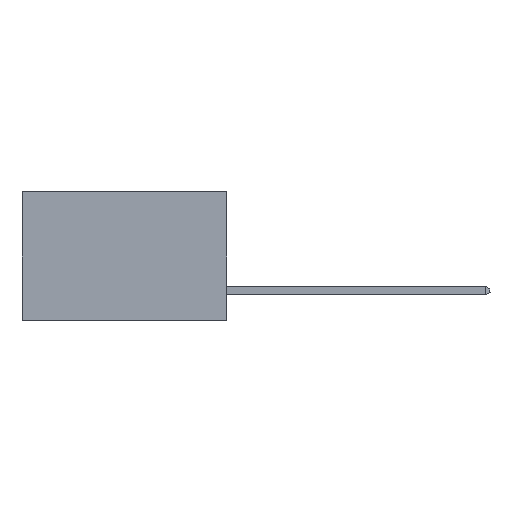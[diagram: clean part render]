
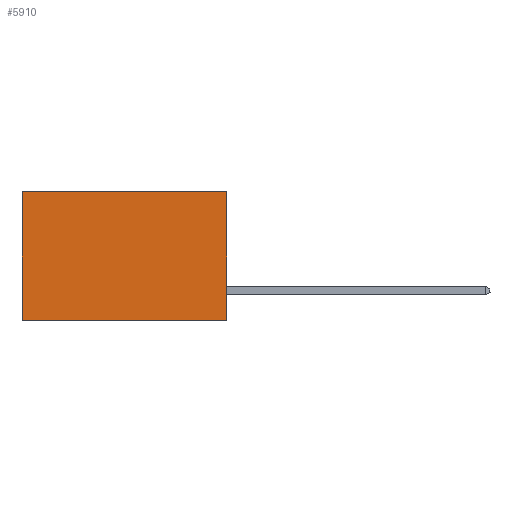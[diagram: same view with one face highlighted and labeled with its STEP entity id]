
A CAD part, left-side view. The second image highlights one B-rep face of the part: STEP entity #5910.
In plain terms, the highlighted planar face has unit normal (-1, 0, 0).
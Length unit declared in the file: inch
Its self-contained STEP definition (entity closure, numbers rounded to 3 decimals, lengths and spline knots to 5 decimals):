
#263 = VECTOR ( 'NONE', #3814, 39.37008 ) ;
#503 = ORIENTED_EDGE ( 'NONE', *, *, #1206, .F. ) ;
#1206 = EDGE_CURVE ( 'NONE', #12290, #2873, #11552, .T. ) ;
#2240 = DIRECTION ( 'NONE',  ( 0., 1., 0. ) ) ;
#2261 = ORIENTED_EDGE ( 'NONE', *, *, #11268, .T. ) ;
#2336 = CARTESIAN_POINT ( 'NONE',  ( 0.277, 0., -0.37 ) ) ;
#2689 = FACE_OUTER_BOUND ( 'NONE', #3065, .T. ) ;
#2873 = VERTEX_POINT ( 'NONE', #12053 ) ;
#3065 = EDGE_LOOP ( 'NONE', ( #5986, #12713, #503, #2261 ) ) ;
#3514 = AXIS2_PLACEMENT_3D ( 'NONE', #10874, #10737, #10732 ) ;
#3814 = DIRECTION ( 'NONE',  ( 0., 0., -1. ) ) ;
#4803 = CARTESIAN_POINT ( 'NONE',  ( 0.277, 0.59, -0.37 ) ) ;
#5076 = VERTEX_POINT ( 'NONE', #17760 ) ;
#5910 = ADVANCED_FACE ( 'NONE', ( #2689 ), #10773, .F. ) ;
#5974 = VERTEX_POINT ( 'NONE', #10279 ) ;
#5986 = ORIENTED_EDGE ( 'NONE', *, *, #9120, .T. ) ;
#7712 = VECTOR ( 'NONE', #8869, 39.37008 ) ;
#8869 = DIRECTION ( 'NONE',  ( 0., 1., 0. ) ) ;
#9120 = EDGE_CURVE ( 'NONE', #5974, #5076, #9216, .T. ) ;
#9216 = LINE ( 'NONE', #4803, #263 ) ;
#9288 = CARTESIAN_POINT ( 'NONE',  ( 0.277, 0., -0.37 ) ) ;
#10261 = DIRECTION ( 'NONE',  ( 0., 0., -1. ) ) ;
#10279 = CARTESIAN_POINT ( 'NONE',  ( 0.277, 0.59, 0. ) ) ;
#10629 = EDGE_CURVE ( 'NONE', #2873, #5076, #14122, .T. ) ;
#10732 = DIRECTION ( 'NONE',  ( 0., 0., -1. ) ) ;
#10737 = DIRECTION ( 'NONE',  ( 1., 0., 0. ) ) ;
#10773 = PLANE ( 'NONE',  #3514 ) ;
#10874 = CARTESIAN_POINT ( 'NONE',  ( 0.277, 0., -0.37 ) ) ;
#11049 = VECTOR ( 'NONE', #10261, 39.37008 ) ;
#11268 = EDGE_CURVE ( 'NONE', #12290, #5974, #19726, .T. ) ;
#11552 = LINE ( 'NONE', #9288, #11049 ) ;
#12053 = CARTESIAN_POINT ( 'NONE',  ( 0.277, 0., -0.37 ) ) ;
#12290 = VERTEX_POINT ( 'NONE', #12760 ) ;
#12713 = ORIENTED_EDGE ( 'NONE', *, *, #10629, .F. ) ;
#12760 = CARTESIAN_POINT ( 'NONE',  ( 0.277, 0., 0. ) ) ;
#14122 = LINE ( 'NONE', #2336, #18100 ) ;
#14952 = CARTESIAN_POINT ( 'NONE',  ( 0.277, 0., 0. ) ) ;
#17760 = CARTESIAN_POINT ( 'NONE',  ( 0.277, 0.59, -0.37 ) ) ;
#18100 = VECTOR ( 'NONE', #2240, 39.37008 ) ;
#19726 = LINE ( 'NONE', #14952, #7712 ) ;
